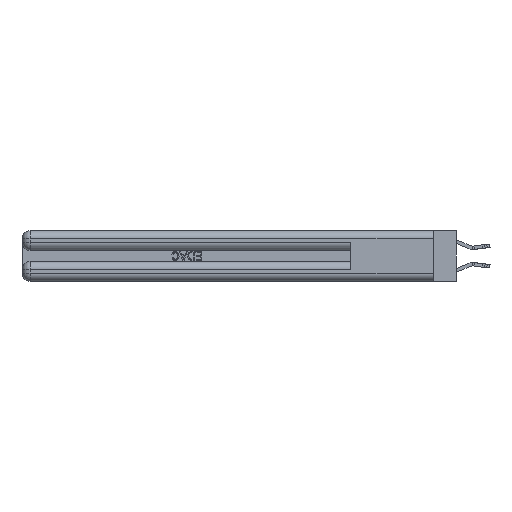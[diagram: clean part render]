
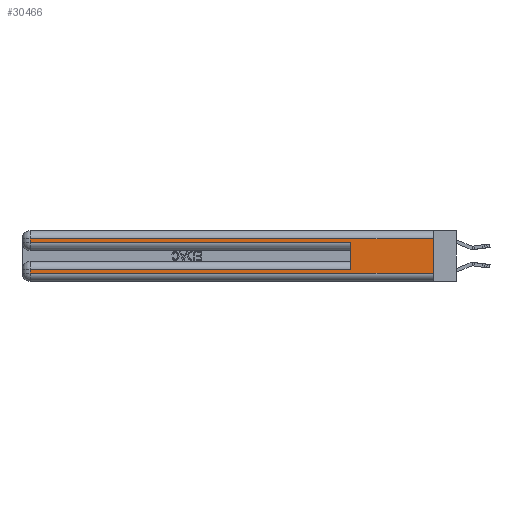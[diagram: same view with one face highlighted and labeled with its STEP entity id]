
A CAD part, left-side view. The second image highlights one B-rep face of the part: STEP entity #30466.
In plain terms, the highlighted planar face has unit normal (-1, 0, 0).
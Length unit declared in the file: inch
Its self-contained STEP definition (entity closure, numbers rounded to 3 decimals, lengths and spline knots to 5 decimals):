
#28 = DIRECTION ( 'NONE',  ( 0., 1., 0. ) ) ;
#1568 = CARTESIAN_POINT ( 'NONE',  ( 0., 0.6, 0.285 ) ) ;
#2126 = DIRECTION ( 'NONE',  ( 0., 0., -1. ) ) ;
#2534 = DIRECTION ( 'NONE',  ( 0., 0., -1. ) ) ;
#2819 = CARTESIAN_POINT ( 'NONE',  ( 0., 0., 0.085 ) ) ;
#3227 = VERTEX_POINT ( 'NONE', #23624 ) ;
#3857 = ORIENTED_EDGE ( 'NONE', *, *, #20576, .T. ) ;
#4320 = CARTESIAN_POINT ( 'NONE',  ( 0., 0., 0.31 ) ) ;
#4667 = FACE_OUTER_BOUND ( 'NONE', #9141, .T. ) ;
#5007 = DIRECTION ( 'NONE',  ( 1., 0., 0. ) ) ;
#5308 = VECTOR ( 'NONE', #14748, 39.37008 ) ;
#6140 = CARTESIAN_POINT ( 'NONE',  ( 0., 2.94, 0.31 ) ) ;
#6278 = VECTOR ( 'NONE', #25285, 39.37008 ) ;
#6844 = DIRECTION ( 'NONE',  ( 0., 0., -1. ) ) ;
#7089 = AXIS2_PLACEMENT_3D ( 'NONE', #20625, #5007, #2534 ) ;
#7179 = LINE ( 'NONE', #9478, #15415 ) ;
#7225 = LINE ( 'NONE', #22378, #10139 ) ;
#7229 = LINE ( 'NONE', #12506, #25265 ) ;
#7748 = LINE ( 'NONE', #2819, #10109 ) ;
#7774 = ORIENTED_EDGE ( 'NONE', *, *, #28263, .T. ) ;
#8778 = EDGE_CURVE ( 'NONE', #16041, #21540, #32361, .T. ) ;
#9033 = DIRECTION ( 'NONE',  ( 0., 0., -1. ) ) ;
#9141 = EDGE_LOOP ( 'NONE', ( #26638, #16965, #3857, #19321, #14202, #21659, #7774, #15295 ) ) ;
#9478 = CARTESIAN_POINT ( 'NONE',  ( 0., 0., 0.37 ) ) ;
#10109 = VECTOR ( 'NONE', #28, 39.37008 ) ;
#10139 = VECTOR ( 'NONE', #12343, 39.37008 ) ;
#10214 = VECTOR ( 'NONE', #13859, 39.37008 ) ;
#11311 = VERTEX_POINT ( 'NONE', #15911 ) ;
#11893 = VERTEX_POINT ( 'NONE', #26392 ) ;
#12343 = DIRECTION ( 'NONE',  ( 0., 1., 0. ) ) ;
#12506 = CARTESIAN_POINT ( 'NONE',  ( 0., 2.94, 0.37 ) ) ;
#12775 = EDGE_CURVE ( 'NONE', #11893, #21540, #29243, .T. ) ;
#13743 = EDGE_CURVE ( 'NONE', #11893, #11311, #7748, .T. ) ;
#13818 = CARTESIAN_POINT ( 'NONE',  ( 0., 0., 0.06 ) ) ;
#13859 = DIRECTION ( 'NONE',  ( 0., -1., 0. ) ) ;
#14202 = ORIENTED_EDGE ( 'NONE', *, *, #12775, .F. ) ;
#14229 = EDGE_CURVE ( 'NONE', #16660, #17625, #7225, .T. ) ;
#14748 = DIRECTION ( 'NONE',  ( 0., 0., 1. ) ) ;
#15295 = ORIENTED_EDGE ( 'NONE', *, *, #24594, .T. ) ;
#15415 = VECTOR ( 'NONE', #6844, 39.37008 ) ;
#15911 = CARTESIAN_POINT ( 'NONE',  ( 0., 2.94, 0.085 ) ) ;
#16041 = VERTEX_POINT ( 'NONE', #28873 ) ;
#16308 = LINE ( 'NONE', #21581, #10214 ) ;
#16660 = VERTEX_POINT ( 'NONE', #4320 ) ;
#16965 = ORIENTED_EDGE ( 'NONE', *, *, #14229, .T. ) ;
#17625 = VERTEX_POINT ( 'NONE', #6140 ) ;
#19072 = VECTOR ( 'NONE', #9033, 39.37008 ) ;
#19321 = ORIENTED_EDGE ( 'NONE', *, *, #8778, .T. ) ;
#20576 = EDGE_CURVE ( 'NONE', #17625, #16041, #7229, .T. ) ;
#20625 = CARTESIAN_POINT ( 'NONE',  ( 0., 0., 0.37 ) ) ;
#21540 = VERTEX_POINT ( 'NONE', #1568 ) ;
#21581 = CARTESIAN_POINT ( 'NONE',  ( 0., 0., 0.06 ) ) ;
#21659 = ORIENTED_EDGE ( 'NONE', *, *, #13743, .T. ) ;
#22348 = CARTESIAN_POINT ( 'NONE',  ( 0., 0., 0.285 ) ) ;
#22378 = CARTESIAN_POINT ( 'NONE',  ( 0., 0., 0.31 ) ) ;
#23534 = CARTESIAN_POINT ( 'NONE',  ( 0., 2.94, 0.37 ) ) ;
#23624 = CARTESIAN_POINT ( 'NONE',  ( 0., 2.94, 0.06 ) ) ;
#24594 = EDGE_CURVE ( 'NONE', #3227, #28210, #16308, .T. ) ;
#24741 = PLANE ( 'NONE',  #7089 ) ;
#25265 = VECTOR ( 'NONE', #2126, 39.37008 ) ;
#25285 = DIRECTION ( 'NONE',  ( 0., -1., 0. ) ) ;
#25994 = LINE ( 'NONE', #23534, #19072 ) ;
#26392 = CARTESIAN_POINT ( 'NONE',  ( 0., 0.6, 0.085 ) ) ;
#26638 = ORIENTED_EDGE ( 'NONE', *, *, #28791, .F. ) ;
#27097 = CARTESIAN_POINT ( 'NONE',  ( 0., 0.6, 0.145 ) ) ;
#28210 = VERTEX_POINT ( 'NONE', #13818 ) ;
#28263 = EDGE_CURVE ( 'NONE', #11311, #3227, #25994, .T. ) ;
#28791 = EDGE_CURVE ( 'NONE', #16660, #28210, #7179, .T. ) ;
#28873 = CARTESIAN_POINT ( 'NONE',  ( 0., 2.94, 0.285 ) ) ;
#29243 = LINE ( 'NONE', #27097, #5308 ) ;
#30466 = ADVANCED_FACE ( 'NONE', ( #4667 ), #24741, .F. ) ;
#32361 = LINE ( 'NONE', #22348, #6278 ) ;
